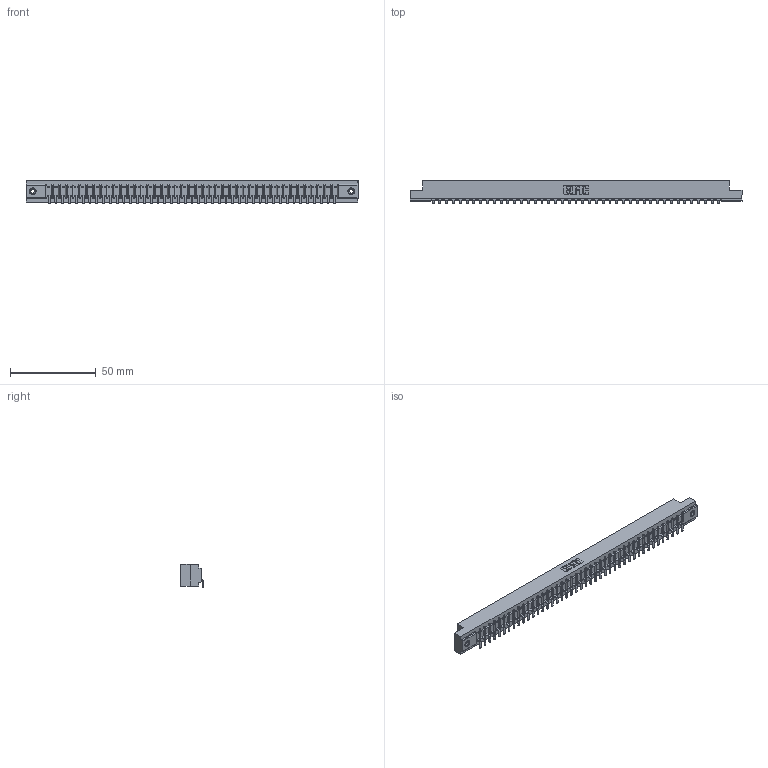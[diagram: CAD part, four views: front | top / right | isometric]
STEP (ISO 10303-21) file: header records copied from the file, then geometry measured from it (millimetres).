
FILE_DESCRIPTION (( 'STEP AP203' ), '1' );
FILE_NAME ('357-043-453-108.STEP', '2020-10-03T13:36:51', ( '' ), ( '' ), 'SwSTEP 2.0', 'SolidWorks 2020', '' );
FILE_SCHEMA (( 'CONFIG_CONTROL_DESIGN' ));
Length unit declared in the file: inch
Products named in the file (4): 307 Part_.156 Dia Mounting Holes; 357-043-453-108; 345-250-001_345-250-003-102; 307-290-002_553
Assembly tree (46 placements, depth 2):
  357-043-453-108
    307 Part_.156 Dia Mounting Holes
    307-290-002_553  x43
    345-250-001_345-250-003-102  x2
Bounding box: 193.4 x 13.32 x 13.5 mm (x, y, z)
Volume: 20696.5 mm3; surface area: 26057.2 mm2
Topology: 46 solids, 46 shells, 3576 faces, 10951 edges, 7174 vertices
Faces by surface type: plane 2123, cylinder 1349, sphere 88, cone 12, torus 4
Entity records: 38779 total; most frequent: CARTESIAN_POINT 6523, ORIENTED_EDGE 6506, DIRECTION 6347, EDGE_CURVE 3253, LINE 2491, VECTOR 2491, VERTEX_POINT 2104, AXIS2_PLACEMENT_3D 1928
